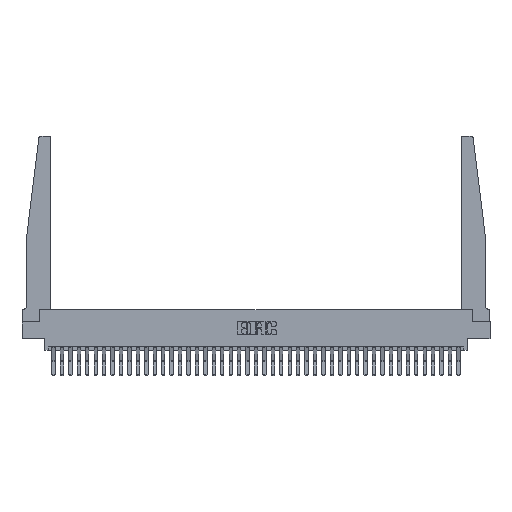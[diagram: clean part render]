
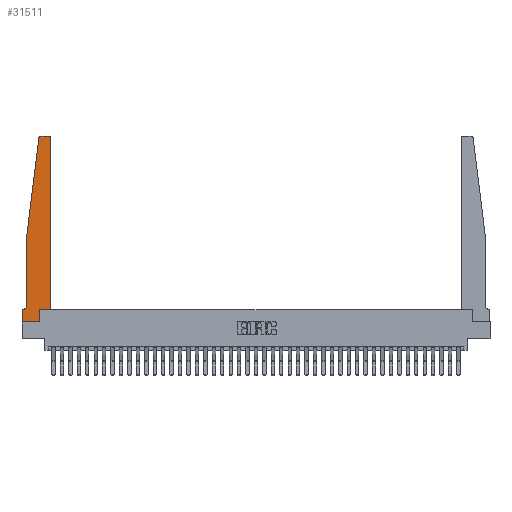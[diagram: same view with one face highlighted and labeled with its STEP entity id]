
A CAD part, top view. The second image highlights one B-rep face of the part: STEP entity #31511.
In plain terms, the highlighted planar face has unit normal (0, 0, 1).
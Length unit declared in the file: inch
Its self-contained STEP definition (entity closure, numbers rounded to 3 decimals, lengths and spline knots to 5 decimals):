
#81 = AXIS2_PLACEMENT_3D ( 'NONE', #31832, #15403, #3572 ) ;
#155 = CARTESIAN_POINT ( 'NONE',  ( 0.2605, 0., 0.37 ) ) ;
#347 = VECTOR ( 'NONE', #24823, 39.37008 ) ;
#403 = CARTESIAN_POINT ( 'NONE',  ( 0.24675, 2.72367, 0.37 ) ) ;
#569 = CIRCLE ( 'NONE', #15328, 0.05 ) ;
#845 = VECTOR ( 'NONE', #23008, 39.37008 ) ;
#1526 = ORIENTED_EDGE ( 'NONE', *, *, #7846, .T. ) ;
#1718 = CARTESIAN_POINT ( 'NONE',  ( 0.2605, 0.18, 0.37 ) ) ;
#2284 = CARTESIAN_POINT ( 'NONE',  ( 0.425, 0.18, 0.37 ) ) ;
#2983 = CARTESIAN_POINT ( 'NONE',  ( 0.015, 0.1875, 0.37 ) ) ;
#3052 = AXIS2_PLACEMENT_3D ( 'NONE', #5060, #24468, #27232 ) ;
#3367 = VERTEX_POINT ( 'NONE', #155 ) ;
#3572 = DIRECTION ( 'NONE',  ( 1., 0., 0. ) ) ;
#4629 = ORIENTED_EDGE ( 'NONE', *, *, #10810, .T. ) ;
#4690 = ORIENTED_EDGE ( 'NONE', *, *, #13150, .T. ) ;
#4697 = FACE_OUTER_BOUND ( 'NONE', #8150, .T. ) ;
#5060 = CARTESIAN_POINT ( 'NONE',  ( 0., 0.1875, 0.37 ) ) ;
#5097 = DIRECTION ( 'NONE',  ( 0., -1., 0. ) ) ;
#5189 = ORIENTED_EDGE ( 'NONE', *, *, #15592, .T. ) ;
#5333 = CARTESIAN_POINT ( 'NONE',  ( 0.065, 1.25, 0.37 ) ) ;
#5404 = CARTESIAN_POINT ( 'NONE',  ( 0.015, 0.2375, 0.37 ) ) ;
#5676 = CARTESIAN_POINT ( 'NONE',  ( 0.065, 0.1875, 0.37 ) ) ;
#6935 = CARTESIAN_POINT ( 'NONE',  ( 0.27653, 2.72, 0.37 ) ) ;
#7151 = CIRCLE ( 'NONE', #81, 0.03 ) ;
#7846 = EDGE_CURVE ( 'NONE', #12939, #35009, #25586, .T. ) ;
#8150 = EDGE_LOOP ( 'NONE', ( #1526, #28925, #5189, #16262, #12123, #25442, #4629, #16714, #15942, #26501, #4690, #22770 ) ) ;
#8172 = DIRECTION ( 'NONE',  ( 0., 0., -1. ) ) ;
#8359 = CIRCLE ( 'NONE', #34310, 0.03 ) ;
#8431 = DIRECTION ( 'NONE',  ( 0., -1., 0. ) ) ;
#8745 = VERTEX_POINT ( 'NONE', #34747 ) ;
#10810 = EDGE_CURVE ( 'NONE', #35702, #20416, #25262, .T. ) ;
#11455 = DIRECTION ( 'NONE',  ( 1., 0., 0. ) ) ;
#11745 = CARTESIAN_POINT ( 'NONE',  ( 0.25, 2.75, 0.37 ) ) ;
#12123 = ORIENTED_EDGE ( 'NONE', *, *, #33635, .T. ) ;
#12523 = DIRECTION ( 'NONE',  ( -0.122, -0.992, 0. ) ) ;
#12939 = VERTEX_POINT ( 'NONE', #18014 ) ;
#13150 = EDGE_CURVE ( 'NONE', #14395, #8745, #27584, .T. ) ;
#13731 = DIRECTION ( 'NONE',  ( -1., 0., 0. ) ) ;
#13965 = CARTESIAN_POINT ( 'NONE',  ( 0.065, 1.25, 0.37 ) ) ;
#14052 = VECTOR ( 'NONE', #12523, 39.37008 ) ;
#14395 = VERTEX_POINT ( 'NONE', #35918 ) ;
#14781 = CARTESIAN_POINT ( 'NONE',  ( 0., 0.1875, 0.37 ) ) ;
#15185 = VERTEX_POINT ( 'NONE', #5333 ) ;
#15263 = CARTESIAN_POINT ( 'NONE',  ( 0., 0., 0.37 ) ) ;
#15271 = DIRECTION ( 'NONE',  ( 1., 0., 0. ) ) ;
#15328 = AXIS2_PLACEMENT_3D ( 'NONE', #5404, #8172, #13731 ) ;
#15403 = DIRECTION ( 'NONE',  ( 0., 0., 1. ) ) ;
#15592 = EDGE_CURVE ( 'NONE', #35001, #15185, #32263, .T. ) ;
#15890 = CARTESIAN_POINT ( 'NONE',  ( 0.065, 0.2375, 0.37 ) ) ;
#15942 = ORIENTED_EDGE ( 'NONE', *, *, #33151, .T. ) ;
#15990 = PLANE ( 'NONE',  #3052 ) ;
#16262 = ORIENTED_EDGE ( 'NONE', *, *, #36260, .T. ) ;
#16714 = ORIENTED_EDGE ( 'NONE', *, *, #17766, .T. ) ;
#16771 = EDGE_CURVE ( 'NONE', #8745, #12939, #7151, .T. ) ;
#17766 = EDGE_CURVE ( 'NONE', #20416, #3367, #35385, .T. ) ;
#18014 = CARTESIAN_POINT ( 'NONE',  ( 0.395, 2.75, 0.37 ) ) ;
#18244 = DIRECTION ( 'NONE',  ( 0., 0., 1. ) ) ;
#18802 = VERTEX_POINT ( 'NONE', #30821 ) ;
#18850 = EDGE_CURVE ( 'NONE', #35009, #35001, #8359, .T. ) ;
#18963 = VECTOR ( 'NONE', #35012, 39.37008 ) ;
#20416 = VERTEX_POINT ( 'NONE', #34297 ) ;
#20476 = CARTESIAN_POINT ( 'NONE',  ( 0.065, 1.25, 0.37 ) ) ;
#22362 = LINE ( 'NONE', #33618, #29709 ) ;
#22573 = CARTESIAN_POINT ( 'NONE',  ( 0.27653, 2.75, 0.37 ) ) ;
#22770 = ORIENTED_EDGE ( 'NONE', *, *, #16771, .T. ) ;
#23008 = DIRECTION ( 'NONE',  ( -1., 0., 0. ) ) ;
#23819 = VECTOR ( 'NONE', #8431, 39.37008 ) ;
#24253 = LINE ( 'NONE', #1718, #36183 ) ;
#24468 = DIRECTION ( 'NONE',  ( 0., 0., 1. ) ) ;
#24619 = DIRECTION ( 'NONE',  ( 0., 1., 0. ) ) ;
#24823 = DIRECTION ( 'NONE',  ( 0., 1., 0. ) ) ;
#25262 = LINE ( 'NONE', #30427, #23819 ) ;
#25442 = ORIENTED_EDGE ( 'NONE', *, *, #34554, .T. ) ;
#25586 = LINE ( 'NONE', #11745, #845 ) ;
#26501 = ORIENTED_EDGE ( 'NONE', *, *, #35525, .T. ) ;
#27232 = DIRECTION ( 'NONE',  ( 1., 0., 0. ) ) ;
#27584 = LINE ( 'NONE', #2284, #347 ) ;
#28925 = ORIENTED_EDGE ( 'NONE', *, *, #18850, .T. ) ;
#29396 = VERTEX_POINT ( 'NONE', #15890 ) ;
#29709 = VECTOR ( 'NONE', #11455, 39.37008 ) ;
#30427 = CARTESIAN_POINT ( 'NONE',  ( 0., 0., 0.37 ) ) ;
#30821 = CARTESIAN_POINT ( 'NONE',  ( 0.2605, 0.18, 0.37 ) ) ;
#31162 = DIRECTION ( 'NONE',  ( -1., 0., 0. ) ) ;
#31433 = VECTOR ( 'NONE', #31162, 39.37008 ) ;
#31511 = ADVANCED_FACE ( 'NONE', ( #4697 ), #15990, .T. ) ;
#31832 = CARTESIAN_POINT ( 'NONE',  ( 0.395, 2.72, 0.37 ) ) ;
#32263 = LINE ( 'NONE', #20476, #14052 ) ;
#33151 = EDGE_CURVE ( 'NONE', #3367, #18802, #24253, .T. ) ;
#33295 = VECTOR ( 'NONE', #5097, 39.37008 ) ;
#33561 = LINE ( 'NONE', #5676, #31433 ) ;
#33618 = CARTESIAN_POINT ( 'NONE',  ( 0.425, 0.18, 0.37 ) ) ;
#33635 = EDGE_CURVE ( 'NONE', #29396, #33711, #569, .T. ) ;
#33711 = VERTEX_POINT ( 'NONE', #2983 ) ;
#34297 = CARTESIAN_POINT ( 'NONE',  ( 0., 0., 0.37 ) ) ;
#34310 = AXIS2_PLACEMENT_3D ( 'NONE', #6935, #18244, #15271 ) ;
#34554 = EDGE_CURVE ( 'NONE', #33711, #35702, #33561, .T. ) ;
#34747 = CARTESIAN_POINT ( 'NONE',  ( 0.425, 2.72, 0.37 ) ) ;
#35001 = VERTEX_POINT ( 'NONE', #403 ) ;
#35009 = VERTEX_POINT ( 'NONE', #22573 ) ;
#35012 = DIRECTION ( 'NONE',  ( 1., 0., 0. ) ) ;
#35385 = LINE ( 'NONE', #15263, #18963 ) ;
#35525 = EDGE_CURVE ( 'NONE', #18802, #14395, #22362, .T. ) ;
#35576 = LINE ( 'NONE', #13965, #33295 ) ;
#35702 = VERTEX_POINT ( 'NONE', #14781 ) ;
#35918 = CARTESIAN_POINT ( 'NONE',  ( 0.425, 0.18, 0.37 ) ) ;
#36183 = VECTOR ( 'NONE', #24619, 39.37008 ) ;
#36260 = EDGE_CURVE ( 'NONE', #15185, #29396, #35576, .T. ) ;
